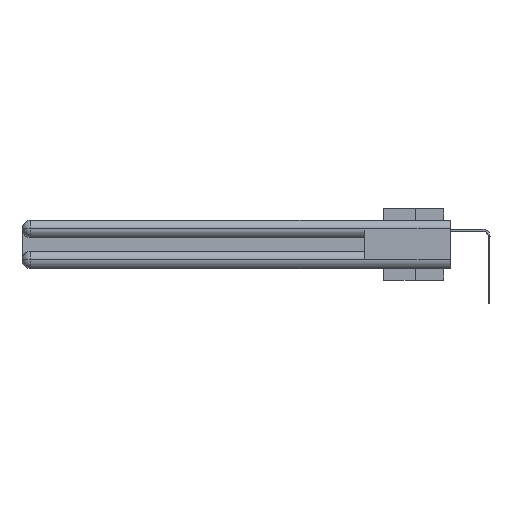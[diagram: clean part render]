
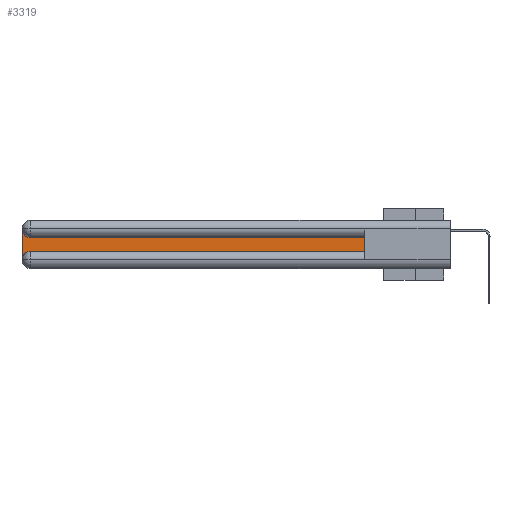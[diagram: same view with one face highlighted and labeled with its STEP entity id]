
A CAD part, left-side view. The second image highlights one B-rep face of the part: STEP entity #3319.
In plain terms, the highlighted planar face has unit normal (-1, 0, 0).
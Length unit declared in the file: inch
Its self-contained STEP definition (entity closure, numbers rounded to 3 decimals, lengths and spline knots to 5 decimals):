
#372 = PLANE ( 'NONE',  #18403 ) ;
#1035 = VECTOR ( 'NONE', #14931, 39.37008 ) ;
#1239 = VERTEX_POINT ( 'NONE', #1469 ) ;
#1258 = CARTESIAN_POINT ( 'NONE',  ( 0.075, 3., -0.2775 ) ) ;
#1469 = CARTESIAN_POINT ( 'NONE',  ( 0.075, 0.6, -0.1225 ) ) ;
#1982 = EDGE_CURVE ( 'NONE', #10112, #17297, #29008, .T. ) ;
#2105 = DIRECTION ( 'NONE',  ( 0., 0., -1. ) ) ;
#3319 = ADVANCED_FACE ( 'NONE', ( #26907 ), #372, .F. ) ;
#3567 = EDGE_CURVE ( 'NONE', #17068, #10112, #26049, .T. ) ;
#3856 = DIRECTION ( 'NONE',  ( 0., 0., -1. ) ) ;
#3977 = CARTESIAN_POINT ( 'NONE',  ( 0.075, 2.94, -0.0625 ) ) ;
#3992 = EDGE_CURVE ( 'NONE', #17297, #11737, #22327, .T. ) ;
#4235 = EDGE_CURVE ( 'NONE', #12947, #1239, #28425, .T. ) ;
#4742 = EDGE_CURVE ( 'NONE', #11737, #12947, #26399, .T. ) ;
#4956 = AXIS2_PLACEMENT_3D ( 'NONE', #3977, #32516, #3856 ) ;
#5862 = CARTESIAN_POINT ( 'NONE',  ( 0.075, 0.6, -0.2175 ) ) ;
#6056 = CARTESIAN_POINT ( 'NONE',  ( 0.075, 0.6, -0.2175 ) ) ;
#6711 = LINE ( 'NONE', #24580, #1035 ) ;
#6903 = CARTESIAN_POINT ( 'NONE',  ( 0.075, 0.6, -0.2175 ) ) ;
#8468 = DIRECTION ( 'NONE',  ( 0., 0., 1. ) ) ;
#9951 = VECTOR ( 'NONE', #2105, 39.37008 ) ;
#9993 = CARTESIAN_POINT ( 'NONE',  ( 0.075, 3., -0.0625 ) ) ;
#10112 = VERTEX_POINT ( 'NONE', #9993 ) ;
#10646 = DIRECTION ( 'NONE',  ( 0., 0., -1. ) ) ;
#11025 = DIRECTION ( 'NONE',  ( 0., -1., 0. ) ) ;
#11737 = VERTEX_POINT ( 'NONE', #23888 ) ;
#12947 = VERTEX_POINT ( 'NONE', #6903 ) ;
#12993 = DIRECTION ( 'NONE',  ( 1., 0., 0. ) ) ;
#13171 = ORIENTED_EDGE ( 'NONE', *, *, #29731, .T. ) ;
#13203 = AXIS2_PLACEMENT_3D ( 'NONE', #31254, #12993, #28988 ) ;
#13712 = ORIENTED_EDGE ( 'NONE', *, *, #4742, .T. ) ;
#13907 = ORIENTED_EDGE ( 'NONE', *, *, #4235, .T. ) ;
#14931 = DIRECTION ( 'NONE',  ( 0., 1., 0. ) ) ;
#17068 = VERTEX_POINT ( 'NONE', #23368 ) ;
#17297 = VERTEX_POINT ( 'NONE', #1258 ) ;
#18261 = ORIENTED_EDGE ( 'NONE', *, *, #3992, .T. ) ;
#18403 = AXIS2_PLACEMENT_3D ( 'NONE', #25767, #28471, #10646 ) ;
#21416 = ORIENTED_EDGE ( 'NONE', *, *, #1982, .T. ) ;
#22327 = CIRCLE ( 'NONE', #13203, 0.06 ) ;
#23368 = CARTESIAN_POINT ( 'NONE',  ( 0.075, 2.94, -0.1225 ) ) ;
#23888 = CARTESIAN_POINT ( 'NONE',  ( 0.075, 2.94, -0.2175 ) ) ;
#24580 = CARTESIAN_POINT ( 'NONE',  ( 0.075, 0.6, -0.1225 ) ) ;
#25767 = CARTESIAN_POINT ( 'NONE',  ( 0.075, 3., -0.1225 ) ) ;
#26049 = CIRCLE ( 'NONE', #4956, 0.06 ) ;
#26399 = LINE ( 'NONE', #6056, #30836 ) ;
#26907 = FACE_OUTER_BOUND ( 'NONE', #30878, .T. ) ;
#28425 = LINE ( 'NONE', #5862, #30872 ) ;
#28471 = DIRECTION ( 'NONE',  ( 1., 0., 0. ) ) ;
#28988 = DIRECTION ( 'NONE',  ( 0., 0., -1. ) ) ;
#29008 = LINE ( 'NONE', #31475, #9951 ) ;
#29379 = ORIENTED_EDGE ( 'NONE', *, *, #3567, .T. ) ;
#29731 = EDGE_CURVE ( 'NONE', #1239, #17068, #6711, .T. ) ;
#30836 = VECTOR ( 'NONE', #11025, 39.37008 ) ;
#30872 = VECTOR ( 'NONE', #8468, 39.37008 ) ;
#30878 = EDGE_LOOP ( 'NONE', ( #13171, #29379, #21416, #18261, #13712, #13907 ) ) ;
#31254 = CARTESIAN_POINT ( 'NONE',  ( 0.075, 2.94, -0.2775 ) ) ;
#31475 = CARTESIAN_POINT ( 'NONE',  ( 0.075, 3., -0.2175 ) ) ;
#32516 = DIRECTION ( 'NONE',  ( 1., 0., 0. ) ) ;
